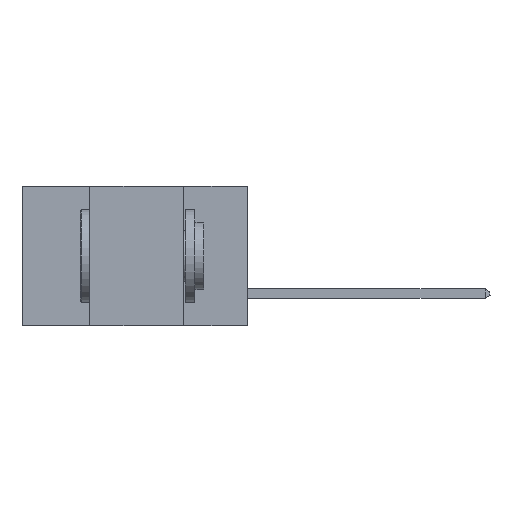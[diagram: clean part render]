
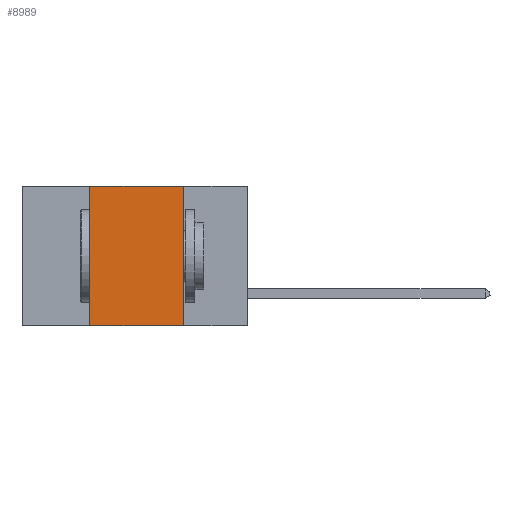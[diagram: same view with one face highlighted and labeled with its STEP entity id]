
A CAD part, left-side view. The second image highlights one B-rep face of the part: STEP entity #8989.
In plain terms, the highlighted planar face has unit normal (-1, 0, 0).
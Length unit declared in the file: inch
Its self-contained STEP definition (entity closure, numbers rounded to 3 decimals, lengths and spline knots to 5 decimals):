
#165 = CARTESIAN_POINT ( 'NONE',  ( 0., 0.6, 0. ) ) ;
#505 = VECTOR ( 'NONE', #2569, 39.37008 ) ;
#661 = CARTESIAN_POINT ( 'NONE',  ( 0., 0.17, -0.37 ) ) ;
#1938 = VECTOR ( 'NONE', #23437, 39.37008 ) ;
#2436 = LINE ( 'NONE', #14762, #12947 ) ;
#2478 = LINE ( 'NONE', #16950, #505 ) ;
#2569 = DIRECTION ( 'NONE',  ( 0., 0., 1. ) ) ;
#4565 = CARTESIAN_POINT ( 'NONE',  ( 0., 0.42, 0. ) ) ;
#4769 = LINE ( 'NONE', #165, #5053 ) ;
#5053 = VECTOR ( 'NONE', #5355, 39.37008 ) ;
#5355 = DIRECTION ( 'NONE',  ( 0., -1., 0. ) ) ;
#5689 = VERTEX_POINT ( 'NONE', #6101 ) ;
#6101 = CARTESIAN_POINT ( 'NONE',  ( 0., 0.17, 0. ) ) ;
#6568 = EDGE_LOOP ( 'NONE', ( #16603, #12430, #17960, #8940 ) ) ;
#6939 = CARTESIAN_POINT ( 'NONE',  ( 0., 0.42, -0.37 ) ) ;
#8513 = DIRECTION ( 'NONE',  ( 1., 0., 0. ) ) ;
#8940 = ORIENTED_EDGE ( 'NONE', *, *, #23031, .T. ) ;
#8989 = ADVANCED_FACE ( 'NONE', ( #19368 ), #16784, .F. ) ;
#9153 = VERTEX_POINT ( 'NONE', #6939 ) ;
#9406 = AXIS2_PLACEMENT_3D ( 'NONE', #13422, #8513, #17365 ) ;
#10576 = CARTESIAN_POINT ( 'NONE',  ( 0., 0.17, 0. ) ) ;
#11972 = VERTEX_POINT ( 'NONE', #661 ) ;
#12221 = EDGE_CURVE ( 'NONE', #9153, #14055, #2478, .T. ) ;
#12323 = EDGE_CURVE ( 'NONE', #5689, #11972, #22862, .T. ) ;
#12430 = ORIENTED_EDGE ( 'NONE', *, *, #22559, .F. ) ;
#12947 = VECTOR ( 'NONE', #22385, 39.37008 ) ;
#13422 = CARTESIAN_POINT ( 'NONE',  ( 0., 0.6, 0. ) ) ;
#14055 = VERTEX_POINT ( 'NONE', #4565 ) ;
#14762 = CARTESIAN_POINT ( 'NONE',  ( 0., 0.6, -0.37 ) ) ;
#16603 = ORIENTED_EDGE ( 'NONE', *, *, #12323, .F. ) ;
#16784 = PLANE ( 'NONE',  #9406 ) ;
#16950 = CARTESIAN_POINT ( 'NONE',  ( 0., 0.42, 0. ) ) ;
#17365 = DIRECTION ( 'NONE',  ( 0., 0., -1. ) ) ;
#17960 = ORIENTED_EDGE ( 'NONE', *, *, #12221, .F. ) ;
#19368 = FACE_OUTER_BOUND ( 'NONE', #6568, .T. ) ;
#22385 = DIRECTION ( 'NONE',  ( 0., -1., 0. ) ) ;
#22559 = EDGE_CURVE ( 'NONE', #14055, #5689, #4769, .T. ) ;
#22862 = LINE ( 'NONE', #10576, #1938 ) ;
#23031 = EDGE_CURVE ( 'NONE', #9153, #11972, #2436, .T. ) ;
#23437 = DIRECTION ( 'NONE',  ( 0., 0., -1. ) ) ;
